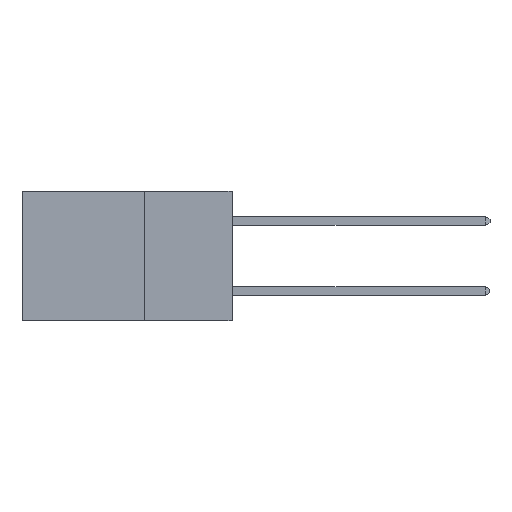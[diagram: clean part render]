
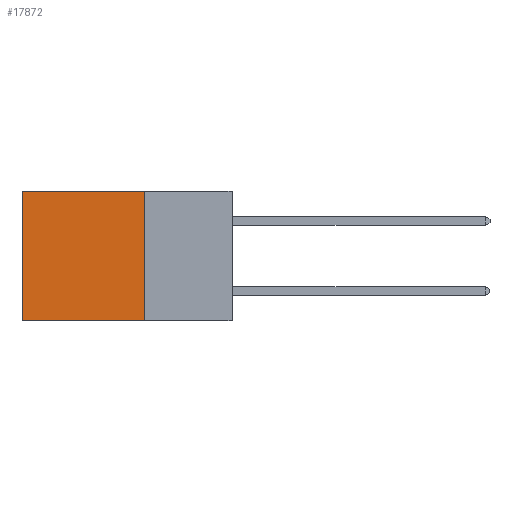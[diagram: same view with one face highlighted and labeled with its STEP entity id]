
A CAD part, left-side view. The second image highlights one B-rep face of the part: STEP entity #17872.
In plain terms, the highlighted planar face has unit normal (-1, 0, 0).
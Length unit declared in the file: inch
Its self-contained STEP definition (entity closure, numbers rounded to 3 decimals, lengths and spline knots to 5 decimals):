
#324 = DIRECTION ( 'NONE',  ( 0., 1., 0. ) ) ;
#510 = FACE_OUTER_BOUND ( 'NONE', #3490, .T. ) ;
#688 = VERTEX_POINT ( 'NONE', #8963 ) ;
#790 = DIRECTION ( 'NONE',  ( 0., 1., 0. ) ) ;
#1768 = LINE ( 'NONE', #18631, #13544 ) ;
#2284 = CARTESIAN_POINT ( 'NONE',  ( 0.2875, 0.25, 0. ) ) ;
#3240 = VECTOR ( 'NONE', #17496, 39.37008 ) ;
#3490 = EDGE_LOOP ( 'NONE', ( #17876, #10698, #14048, #16977 ) ) ;
#4425 = VERTEX_POINT ( 'NONE', #4951 ) ;
#4951 = CARTESIAN_POINT ( 'NONE',  ( 0.2875, 0.25, -0.37 ) ) ;
#5215 = CARTESIAN_POINT ( 'NONE',  ( 0.2875, 0.6, -0.37 ) ) ;
#5301 = DIRECTION ( 'NONE',  ( 0., 0., -1. ) ) ;
#5468 = DIRECTION ( 'NONE',  ( 0., 0., -1. ) ) ;
#6973 = CARTESIAN_POINT ( 'NONE',  ( 0.2875, 0.6, 0. ) ) ;
#7300 = LINE ( 'NONE', #6973, #3240 ) ;
#7903 = LINE ( 'NONE', #14305, #12437 ) ;
#8141 = VERTEX_POINT ( 'NONE', #12531 ) ;
#8963 = CARTESIAN_POINT ( 'NONE',  ( 0.2875, 0.25, 0. ) ) ;
#10133 = VECTOR ( 'NONE', #790, 39.37008 ) ;
#10698 = ORIENTED_EDGE ( 'NONE', *, *, #10932, .F. ) ;
#10932 = EDGE_CURVE ( 'NONE', #4425, #17786, #1768, .T. ) ;
#12158 = EDGE_CURVE ( 'NONE', #8141, #17786, #7300, .T. ) ;
#12437 = VECTOR ( 'NONE', #5301, 39.37008 ) ;
#12531 = CARTESIAN_POINT ( 'NONE',  ( 0.2875, 0.6, 0. ) ) ;
#12994 = PLANE ( 'NONE',  #18810 ) ;
#13544 = VECTOR ( 'NONE', #324, 39.37008 ) ;
#14048 = ORIENTED_EDGE ( 'NONE', *, *, #17075, .F. ) ;
#14053 = EDGE_CURVE ( 'NONE', #688, #8141, #14095, .T. ) ;
#14095 = LINE ( 'NONE', #19055, #10133 ) ;
#14305 = CARTESIAN_POINT ( 'NONE',  ( 0.2875, 0.25, 0. ) ) ;
#14463 = DIRECTION ( 'NONE',  ( 1., 0., 0. ) ) ;
#16977 = ORIENTED_EDGE ( 'NONE', *, *, #14053, .T. ) ;
#17075 = EDGE_CURVE ( 'NONE', #688, #4425, #7903, .T. ) ;
#17496 = DIRECTION ( 'NONE',  ( 0., 0., -1. ) ) ;
#17786 = VERTEX_POINT ( 'NONE', #5215 ) ;
#17872 = ADVANCED_FACE ( 'NONE', ( #510 ), #12994, .F. ) ;
#17876 = ORIENTED_EDGE ( 'NONE', *, *, #12158, .T. ) ;
#18631 = CARTESIAN_POINT ( 'NONE',  ( 0.2875, 0.25, -0.37 ) ) ;
#18810 = AXIS2_PLACEMENT_3D ( 'NONE', #2284, #14463, #5468 ) ;
#19055 = CARTESIAN_POINT ( 'NONE',  ( 0.2875, 0.25, 0. ) ) ;
